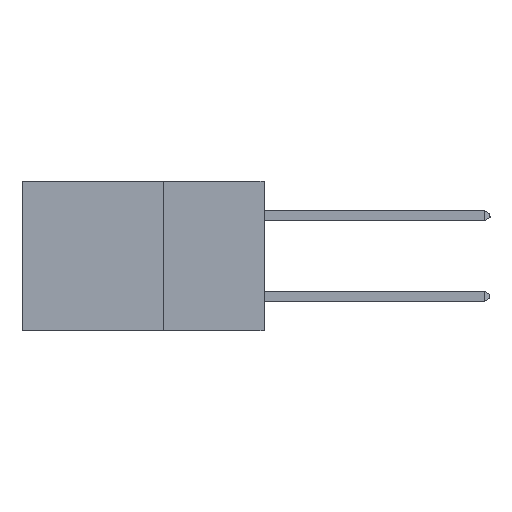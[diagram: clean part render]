
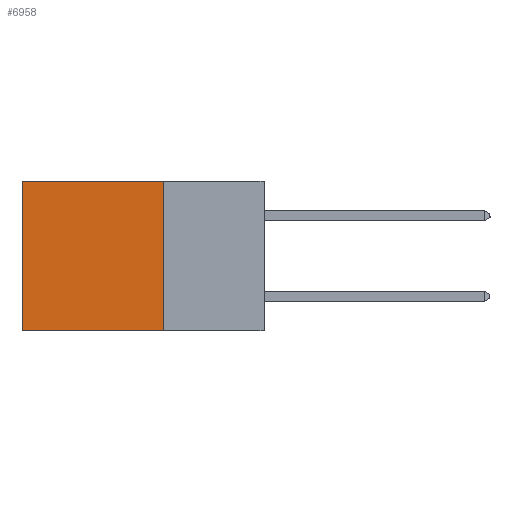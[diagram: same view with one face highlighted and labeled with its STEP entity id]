
A CAD part, left-side view. The second image highlights one B-rep face of the part: STEP entity #6958.
In plain terms, the highlighted planar face has unit normal (-1, 0, 0).
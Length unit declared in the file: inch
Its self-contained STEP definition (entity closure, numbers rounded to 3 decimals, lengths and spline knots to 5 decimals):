
#1383 = FACE_OUTER_BOUND ( 'NONE', #16033, .T. ) ;
#2573 = EDGE_CURVE ( 'NONE', #13552, #19194, #4670, .T. ) ;
#2644 = EDGE_CURVE ( 'NONE', #2912, #13552, #12459, .T. ) ;
#2860 = EDGE_CURVE ( 'NONE', #2912, #7516, #16814, .T. ) ;
#2912 = VERTEX_POINT ( 'NONE', #7499 ) ;
#3981 = CARTESIAN_POINT ( 'NONE',  ( 0.298, 0.25, -0.37 ) ) ;
#4670 = LINE ( 'NONE', #11915, #18172 ) ;
#6711 = PLANE ( 'NONE',  #13316 ) ;
#6958 = ADVANCED_FACE ( 'NONE', ( #1383 ), #6711, .F. ) ;
#7499 = CARTESIAN_POINT ( 'NONE',  ( 0.298, 0.25, 0. ) ) ;
#7516 = VERTEX_POINT ( 'NONE', #18498 ) ;
#8514 = CARTESIAN_POINT ( 'NONE',  ( 0.298, 0.6, 0. ) ) ;
#9892 = ORIENTED_EDGE ( 'NONE', *, *, #2644, .F. ) ;
#9944 = CARTESIAN_POINT ( 'NONE',  ( 0.298, 0.6, -0.37 ) ) ;
#10278 = DIRECTION ( 'NONE',  ( 0., 0., -1. ) ) ;
#11915 = CARTESIAN_POINT ( 'NONE',  ( 0.298, 0.25, -0.37 ) ) ;
#12117 = LINE ( 'NONE', #8514, #12667 ) ;
#12166 = VECTOR ( 'NONE', #16202, 39.37008 ) ;
#12459 = LINE ( 'NONE', #15593, #21168 ) ;
#12667 = VECTOR ( 'NONE', #20731, 39.37008 ) ;
#13316 = AXIS2_PLACEMENT_3D ( 'NONE', #18989, #20729, #10278 ) ;
#13552 = VERTEX_POINT ( 'NONE', #3981 ) ;
#14709 = ORIENTED_EDGE ( 'NONE', *, *, #2573, .F. ) ;
#15366 = DIRECTION ( 'NONE',  ( 0., 1., 0. ) ) ;
#15593 = CARTESIAN_POINT ( 'NONE',  ( 0.298, 0.25, 0. ) ) ;
#16033 = EDGE_LOOP ( 'NONE', ( #18452, #14709, #9892, #20738 ) ) ;
#16202 = DIRECTION ( 'NONE',  ( 0., 1., 0. ) ) ;
#16751 = EDGE_CURVE ( 'NONE', #7516, #19194, #12117, .T. ) ;
#16814 = LINE ( 'NONE', #17846, #12166 ) ;
#17323 = DIRECTION ( 'NONE',  ( 0., 0., -1. ) ) ;
#17846 = CARTESIAN_POINT ( 'NONE',  ( 0.298, 0.25, 0. ) ) ;
#18172 = VECTOR ( 'NONE', #15366, 39.37008 ) ;
#18452 = ORIENTED_EDGE ( 'NONE', *, *, #16751, .T. ) ;
#18498 = CARTESIAN_POINT ( 'NONE',  ( 0.298, 0.6, 0. ) ) ;
#18989 = CARTESIAN_POINT ( 'NONE',  ( 0.298, 0.25, 0. ) ) ;
#19194 = VERTEX_POINT ( 'NONE', #9944 ) ;
#20729 = DIRECTION ( 'NONE',  ( 1., 0., 0. ) ) ;
#20731 = DIRECTION ( 'NONE',  ( 0., 0., -1. ) ) ;
#20738 = ORIENTED_EDGE ( 'NONE', *, *, #2860, .T. ) ;
#21168 = VECTOR ( 'NONE', #17323, 39.37008 ) ;
